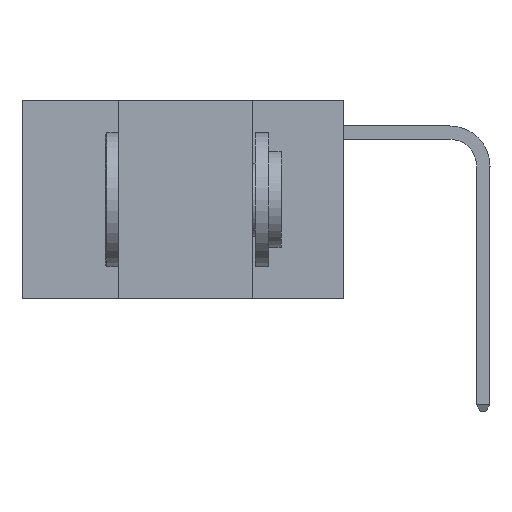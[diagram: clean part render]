
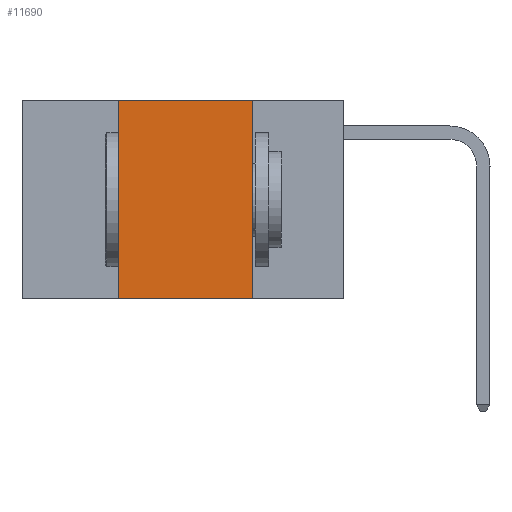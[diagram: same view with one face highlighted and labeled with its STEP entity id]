
A CAD part, left-side view. The second image highlights one B-rep face of the part: STEP entity #11690.
In plain terms, the highlighted planar face has unit normal (-1, 0, 0).
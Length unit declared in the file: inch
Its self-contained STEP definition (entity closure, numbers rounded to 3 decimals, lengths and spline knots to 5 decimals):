
#597 = AXIS2_PLACEMENT_3D ( 'NONE', #1611, #6293, #22130 ) ;
#945 = VECTOR ( 'NONE', #7613, 39.37008 ) ;
#957 = LINE ( 'NONE', #6584, #17626 ) ;
#1087 = CARTESIAN_POINT ( 'NONE',  ( 0., 0.17, -0.37 ) ) ;
#1611 = CARTESIAN_POINT ( 'NONE',  ( 0., 0.6, 0. ) ) ;
#2505 = LINE ( 'NONE', #4769, #24487 ) ;
#2786 = CARTESIAN_POINT ( 'NONE',  ( 0., 0.42, 0. ) ) ;
#4769 = CARTESIAN_POINT ( 'NONE',  ( 0., 0.6, -0.37 ) ) ;
#5158 = ORIENTED_EDGE ( 'NONE', *, *, #5278, .T. ) ;
#5278 = EDGE_CURVE ( 'NONE', #20513, #9261, #2505, .T. ) ;
#5689 = CARTESIAN_POINT ( 'NONE',  ( 0., 0.42, -0.37 ) ) ;
#6293 = DIRECTION ( 'NONE',  ( 1., 0., 0. ) ) ;
#6584 = CARTESIAN_POINT ( 'NONE',  ( 0., 0.17, 0. ) ) ;
#7096 = DIRECTION ( 'NONE',  ( 0., -1., 0. ) ) ;
#7613 = DIRECTION ( 'NONE',  ( 0., 0., 1. ) ) ;
#8472 = VERTEX_POINT ( 'NONE', #2786 ) ;
#9261 = VERTEX_POINT ( 'NONE', #1087 ) ;
#9859 = EDGE_CURVE ( 'NONE', #20513, #8472, #25756, .T. ) ;
#11690 = ADVANCED_FACE ( 'NONE', ( #19342 ), #13038, .F. ) ;
#12312 = CARTESIAN_POINT ( 'NONE',  ( 0., 0.17, 0. ) ) ;
#12396 = LINE ( 'NONE', #29016, #18385 ) ;
#12927 = EDGE_LOOP ( 'NONE', ( #22238, #14421, #27294, #5158 ) ) ;
#13038 = PLANE ( 'NONE',  #597 ) ;
#14421 = ORIENTED_EDGE ( 'NONE', *, *, #15131, .F. ) ;
#15131 = EDGE_CURVE ( 'NONE', #8472, #16875, #12396, .T. ) ;
#16604 = CARTESIAN_POINT ( 'NONE',  ( 0., 0.42, 0. ) ) ;
#16875 = VERTEX_POINT ( 'NONE', #12312 ) ;
#17626 = VECTOR ( 'NONE', #29124, 39.37008 ) ;
#18385 = VECTOR ( 'NONE', #24480, 39.37008 ) ;
#19342 = FACE_OUTER_BOUND ( 'NONE', #12927, .T. ) ;
#20513 = VERTEX_POINT ( 'NONE', #5689 ) ;
#22130 = DIRECTION ( 'NONE',  ( 0., 0., -1. ) ) ;
#22238 = ORIENTED_EDGE ( 'NONE', *, *, #28626, .F. ) ;
#24480 = DIRECTION ( 'NONE',  ( 0., -1., 0. ) ) ;
#24487 = VECTOR ( 'NONE', #7096, 39.37008 ) ;
#25756 = LINE ( 'NONE', #16604, #945 ) ;
#27294 = ORIENTED_EDGE ( 'NONE', *, *, #9859, .F. ) ;
#28626 = EDGE_CURVE ( 'NONE', #16875, #9261, #957, .T. ) ;
#29016 = CARTESIAN_POINT ( 'NONE',  ( 0., 0.6, 0. ) ) ;
#29124 = DIRECTION ( 'NONE',  ( 0., 0., -1. ) ) ;
